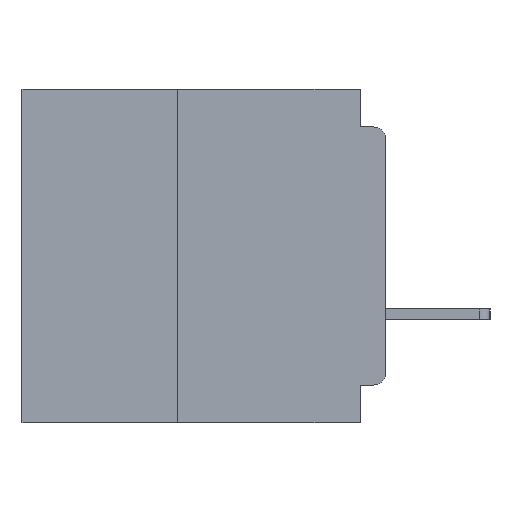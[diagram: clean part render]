
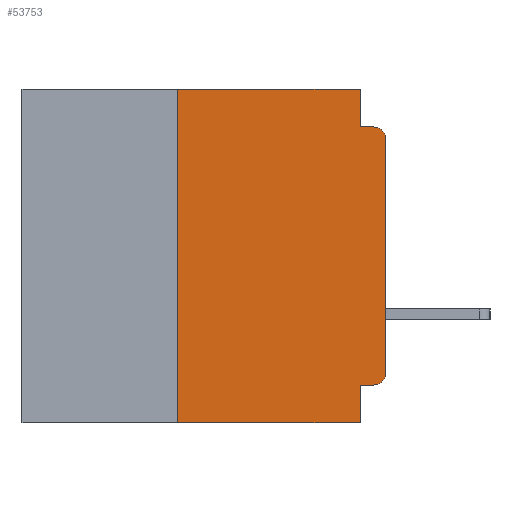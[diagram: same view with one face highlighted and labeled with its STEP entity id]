
A CAD part, left-side view. The second image highlights one B-rep face of the part: STEP entity #53753.
In plain terms, the highlighted planar face has unit normal (-1, 0, 0).
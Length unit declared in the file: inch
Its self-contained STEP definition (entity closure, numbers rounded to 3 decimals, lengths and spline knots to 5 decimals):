
#676 = ORIENTED_EDGE ( 'NONE', *, *, #29920, .F. ) ;
#2310 = LINE ( 'NONE', #30115, #39958 ) ;
#2514 = VERTEX_POINT ( 'NONE', #39317 ) ;
#3899 = CARTESIAN_POINT ( 'NONE',  ( 0., 0., -0.045 ) ) ;
#4340 = EDGE_CURVE ( 'NONE', #7235, #6255, #30026, .T. ) ;
#4481 = VECTOR ( 'NONE', #28871, 39.37008 ) ;
#5093 = DIRECTION ( 'NONE',  ( 1., 0., 0. ) ) ;
#5193 = VECTOR ( 'NONE', #61303, 39.37008 ) ;
#5603 = ORIENTED_EDGE ( 'NONE', *, *, #25290, .F. ) ;
#5657 = DIRECTION ( 'NONE',  ( 0., 0., 1. ) ) ;
#5887 = VERTEX_POINT ( 'NONE', #56025 ) ;
#6255 = VERTEX_POINT ( 'NONE', #44243 ) ;
#6427 = EDGE_CURVE ( 'NONE', #6255, #59234, #52801, .T. ) ;
#7235 = VERTEX_POINT ( 'NONE', #17673 ) ;
#8229 = VERTEX_POINT ( 'NONE', #23609 ) ;
#8749 = DIRECTION ( 'NONE',  ( 0., -1., 0. ) ) ;
#11193 = CARTESIAN_POINT ( 'NONE',  ( 0., 0.031, -0.4 ) ) ;
#13797 = CARTESIAN_POINT ( 'NONE',  ( 0., 0.031, 0. ) ) ;
#15268 = DIRECTION ( 'NONE',  ( -1., 0., 0. ) ) ;
#16965 = CARTESIAN_POINT ( 'NONE',  ( 0., 0.25, -0.4 ) ) ;
#17673 = CARTESIAN_POINT ( 'NONE',  ( 0., 0.015, -0.355 ) ) ;
#17993 = VERTEX_POINT ( 'NONE', #46354 ) ;
#18541 = CARTESIAN_POINT ( 'NONE',  ( 0., 0.015, -0.06 ) ) ;
#19397 = VERTEX_POINT ( 'NONE', #16965 ) ;
#19426 = EDGE_CURVE ( 'NONE', #36824, #54340, #44361, .T. ) ;
#21158 = ORIENTED_EDGE ( 'NONE', *, *, #6427, .F. ) ;
#21633 = LINE ( 'NONE', #3899, #34748 ) ;
#21700 = DIRECTION ( 'NONE',  ( 0., -1., 0. ) ) ;
#22103 = VECTOR ( 'NONE', #54148, 39.37008 ) ;
#23422 = DIRECTION ( 'NONE',  ( 0., 0., -1. ) ) ;
#23609 = CARTESIAN_POINT ( 'NONE',  ( 0., 0.031, -0.045 ) ) ;
#25290 = EDGE_CURVE ( 'NONE', #19397, #5887, #2310, .T. ) ;
#26347 = EDGE_CURVE ( 'NONE', #17993, #8229, #32138, .T. ) ;
#28871 = DIRECTION ( 'NONE',  ( 0., 0., -1. ) ) ;
#28983 = AXIS2_PLACEMENT_3D ( 'NONE', #44725, #15268, #49650 ) ;
#29063 = ORIENTED_EDGE ( 'NONE', *, *, #52204, .F. ) ;
#29920 = EDGE_CURVE ( 'NONE', #5887, #17993, #31917, .T. ) ;
#30026 = LINE ( 'NONE', #43097, #31596 ) ;
#30115 = CARTESIAN_POINT ( 'NONE',  ( 0., 0.25, -0.4 ) ) ;
#30369 = VECTOR ( 'NONE', #21700, 39.37008 ) ;
#30545 = EDGE_LOOP ( 'NONE', ( #41868, #55239, #29063, #60879, #676, #5603, #43442, #21158, #38612, #44967 ) ) ;
#31596 = VECTOR ( 'NONE', #42822, 39.37008 ) ;
#31917 = LINE ( 'NONE', #60501, #30369 ) ;
#31988 = AXIS2_PLACEMENT_3D ( 'NONE', #18541, #52894, #23422 ) ;
#32042 = CARTESIAN_POINT ( 'NONE',  ( 0., 0., 0. ) ) ;
#32138 = LINE ( 'NONE', #13797, #4481 ) ;
#32326 = CIRCLE ( 'NONE', #28983, 0.015 ) ;
#34493 = PLANE ( 'NONE',  #34565 ) ;
#34565 = AXIS2_PLACEMENT_3D ( 'NONE', #43932, #5093, #39423 ) ;
#34748 = VECTOR ( 'NONE', #8749, 39.37008 ) ;
#35644 = DIRECTION ( 'NONE',  ( 0., 0., -1. ) ) ;
#36481 = EDGE_CURVE ( 'NONE', #54340, #2514, #60497, .T. ) ;
#36666 = EDGE_CURVE ( 'NONE', #19397, #59234, #61225, .T. ) ;
#36824 = VERTEX_POINT ( 'NONE', #61158 ) ;
#38245 = VECTOR ( 'NONE', #35644, 39.37008 ) ;
#38612 = ORIENTED_EDGE ( 'NONE', *, *, #4340, .F. ) ;
#39317 = CARTESIAN_POINT ( 'NONE',  ( 0., 0.015, -0.045 ) ) ;
#39423 = DIRECTION ( 'NONE',  ( 0., 0., -1. ) ) ;
#39958 = VECTOR ( 'NONE', #5657, 39.37008 ) ;
#41868 = ORIENTED_EDGE ( 'NONE', *, *, #19426, .T. ) ;
#42199 = FACE_OUTER_BOUND ( 'NONE', #30545, .T. ) ;
#42822 = DIRECTION ( 'NONE',  ( 0., 1., 0. ) ) ;
#43097 = CARTESIAN_POINT ( 'NONE',  ( 0., 0., -0.355 ) ) ;
#43442 = ORIENTED_EDGE ( 'NONE', *, *, #36666, .T. ) ;
#43932 = CARTESIAN_POINT ( 'NONE',  ( 0., 0.437, 0. ) ) ;
#44243 = CARTESIAN_POINT ( 'NONE',  ( 0., 0.031, -0.355 ) ) ;
#44361 = LINE ( 'NONE', #32042, #5193 ) ;
#44725 = CARTESIAN_POINT ( 'NONE',  ( 0., 0.015, -0.34 ) ) ;
#44967 = ORIENTED_EDGE ( 'NONE', *, *, #50021, .T. ) ;
#45534 = CARTESIAN_POINT ( 'NONE',  ( 0., 0.031, -0.4 ) ) ;
#46354 = CARTESIAN_POINT ( 'NONE',  ( 0., 0.031, 0. ) ) ;
#49021 = CARTESIAN_POINT ( 'NONE',  ( 0., 0., -0.06 ) ) ;
#49650 = DIRECTION ( 'NONE',  ( 0., 0., -1. ) ) ;
#50021 = EDGE_CURVE ( 'NONE', #7235, #36824, #32326, .T. ) ;
#52204 = EDGE_CURVE ( 'NONE', #8229, #2514, #21633, .T. ) ;
#52801 = LINE ( 'NONE', #45534, #38245 ) ;
#52894 = DIRECTION ( 'NONE',  ( -1., 0., 0. ) ) ;
#53753 = ADVANCED_FACE ( 'NONE', ( #42199 ), #34493, .F. ) ;
#54148 = DIRECTION ( 'NONE',  ( 0., -1., 0. ) ) ;
#54340 = VERTEX_POINT ( 'NONE', #49021 ) ;
#55239 = ORIENTED_EDGE ( 'NONE', *, *, #36481, .T. ) ;
#56025 = CARTESIAN_POINT ( 'NONE',  ( 0., 0.25, 0. ) ) ;
#58827 = CARTESIAN_POINT ( 'NONE',  ( 0., 0.437, -0.4 ) ) ;
#59234 = VERTEX_POINT ( 'NONE', #11193 ) ;
#60497 = CIRCLE ( 'NONE', #31988, 0.015 ) ;
#60501 = CARTESIAN_POINT ( 'NONE',  ( 0., 0.437, 0. ) ) ;
#60879 = ORIENTED_EDGE ( 'NONE', *, *, #26347, .F. ) ;
#61158 = CARTESIAN_POINT ( 'NONE',  ( 0., 0., -0.34 ) ) ;
#61225 = LINE ( 'NONE', #58827, #22103 ) ;
#61303 = DIRECTION ( 'NONE',  ( 0., 0., 1. ) ) ;
